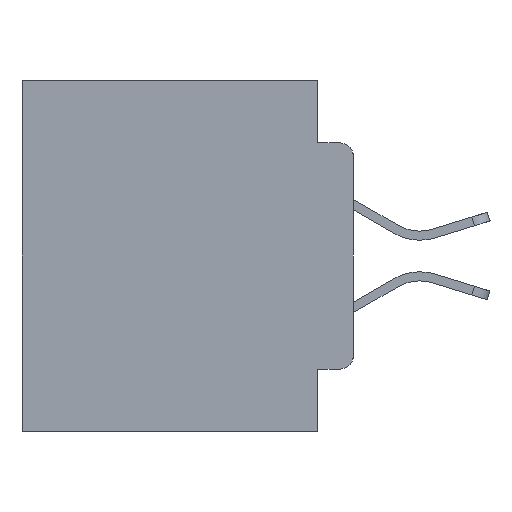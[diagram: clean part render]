
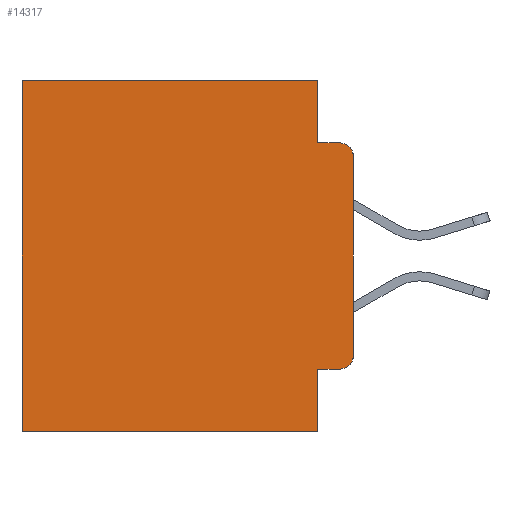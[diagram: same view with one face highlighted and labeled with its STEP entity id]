
A CAD part, left-side view. The second image highlights one B-rep face of the part: STEP entity #14317.
In plain terms, the highlighted planar face has unit normal (-1, 0, 0).
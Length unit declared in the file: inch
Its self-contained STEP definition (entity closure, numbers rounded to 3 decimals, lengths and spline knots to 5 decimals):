
#11 = DIRECTION ( 'NONE',  ( 0., -1., 0. ) ) ;
#180 = EDGE_CURVE ( 'NONE', #10233, #14996, #1160, .T. ) ;
#292 = DIRECTION ( 'NONE',  ( 0., -1., 0. ) ) ;
#867 = LINE ( 'NONE', #10443, #5793 ) ;
#1045 = ORIENTED_EDGE ( 'NONE', *, *, #18575, .F. ) ;
#1160 = LINE ( 'NONE', #14330, #7426 ) ;
#1715 = CARTESIAN_POINT ( 'NONE',  ( 0.298, 0., -0.3915 ) ) ;
#1781 = VECTOR ( 'NONE', #10730, 39.37008 ) ;
#1983 = PLANE ( 'NONE',  #9434 ) ;
#2389 = CARTESIAN_POINT ( 'NONE',  ( 0.298, 0.02, -0.1085 ) ) ;
#2876 = VERTEX_POINT ( 'NONE', #13239 ) ;
#3008 = EDGE_CURVE ( 'NONE', #16063, #8864, #10529, .T. ) ;
#3154 = ORIENTED_EDGE ( 'NONE', *, *, #12785, .F. ) ;
#3588 = AXIS2_PLACEMENT_3D ( 'NONE', #20875, #8948, #22816 ) ;
#4465 = DIRECTION ( 'NONE',  ( 0., 0., -1. ) ) ;
#4980 = LINE ( 'NONE', #25865, #25552 ) ;
#5456 = VERTEX_POINT ( 'NONE', #16748 ) ;
#5793 = VECTOR ( 'NONE', #11, 39.37008 ) ;
#5904 = FACE_OUTER_BOUND ( 'NONE', #18504, .T. ) ;
#6209 = DIRECTION ( 'NONE',  ( 1., 0., 0. ) ) ;
#6647 = CARTESIAN_POINT ( 'NONE',  ( 0.298, 0., -0.1085 ) ) ;
#7142 = ORIENTED_EDGE ( 'NONE', *, *, #14730, .F. ) ;
#7385 = EDGE_CURVE ( 'NONE', #23375, #14602, #9336, .T. ) ;
#7426 = VECTOR ( 'NONE', #9714, 39.37008 ) ;
#7862 = CARTESIAN_POINT ( 'NONE',  ( 0.298, 0.051, 0. ) ) ;
#8667 = CARTESIAN_POINT ( 'NONE',  ( 0.298, 0.051, -0.0885 ) ) ;
#8702 = CARTESIAN_POINT ( 'NONE',  ( 0.298, 0., 0. ) ) ;
#8864 = VERTEX_POINT ( 'NONE', #9341 ) ;
#8948 = DIRECTION ( 'NONE',  ( -1., 0., 0. ) ) ;
#8970 = LINE ( 'NONE', #8667, #19015 ) ;
#9336 = CIRCLE ( 'NONE', #18725, 0.02 ) ;
#9341 = CARTESIAN_POINT ( 'NONE',  ( 0.298, 0.473, -0.5 ) ) ;
#9434 = AXIS2_PLACEMENT_3D ( 'NONE', #18357, #6209, #20303 ) ;
#9667 = ORIENTED_EDGE ( 'NONE', *, *, #20681, .T. ) ;
#9714 = DIRECTION ( 'NONE',  ( 0., 0., -1. ) ) ;
#9991 = EDGE_CURVE ( 'NONE', #2876, #24750, #14282, .T. ) ;
#10041 = ORIENTED_EDGE ( 'NONE', *, *, #9991, .F. ) ;
#10123 = ORIENTED_EDGE ( 'NONE', *, *, #180, .F. ) ;
#10233 = VERTEX_POINT ( 'NONE', #7862 ) ;
#10443 = CARTESIAN_POINT ( 'NONE',  ( 0.298, 0.051, -0.4115 ) ) ;
#10529 = LINE ( 'NONE', #21386, #11164 ) ;
#10730 = DIRECTION ( 'NONE',  ( 0., 1., 0. ) ) ;
#11164 = VECTOR ( 'NONE', #14264, 39.37008 ) ;
#12785 = EDGE_CURVE ( 'NONE', #24750, #8864, #4980, .T. ) ;
#13239 = CARTESIAN_POINT ( 'NONE',  ( 0.298, 0.051, -0.4115 ) ) ;
#13597 = ORIENTED_EDGE ( 'NONE', *, *, #16756, .T. ) ;
#14264 = DIRECTION ( 'NONE',  ( 0., 0., -1. ) ) ;
#14282 = LINE ( 'NONE', #14794, #18316 ) ;
#14317 = ADVANCED_FACE ( 'NONE', ( #5904 ), #1983, .F. ) ;
#14330 = CARTESIAN_POINT ( 'NONE',  ( 0.298, 0.051, 0. ) ) ;
#14602 = VERTEX_POINT ( 'NONE', #23064 ) ;
#14730 = EDGE_CURVE ( 'NONE', #23375, #16025, #17338, .T. ) ;
#14794 = CARTESIAN_POINT ( 'NONE',  ( 0.298, 0.051, 0. ) ) ;
#14996 = VERTEX_POINT ( 'NONE', #25937 ) ;
#15062 = CARTESIAN_POINT ( 'NONE',  ( 0.298, 0.051, -0.5 ) ) ;
#15657 = CARTESIAN_POINT ( 'NONE',  ( 0.298, 0., 0. ) ) ;
#16025 = VERTEX_POINT ( 'NONE', #1715 ) ;
#16063 = VERTEX_POINT ( 'NONE', #18101 ) ;
#16729 = VECTOR ( 'NONE', #25299, 39.37008 ) ;
#16748 = CARTESIAN_POINT ( 'NONE',  ( 0.298, 0.02, -0.4115 ) ) ;
#16754 = DIRECTION ( 'NONE',  ( -1., 0., 0. ) ) ;
#16756 = EDGE_CURVE ( 'NONE', #2876, #5456, #867, .T. ) ;
#17338 = LINE ( 'NONE', #15657, #16729 ) ;
#17623 = ORIENTED_EDGE ( 'NONE', *, *, #7385, .T. ) ;
#17948 = EDGE_CURVE ( 'NONE', #10233, #16063, #18244, .T. ) ;
#18101 = CARTESIAN_POINT ( 'NONE',  ( 0.298, 0.473, 0. ) ) ;
#18243 = DIRECTION ( 'NONE',  ( 0., 1., 0. ) ) ;
#18244 = LINE ( 'NONE', #8702, #1781 ) ;
#18316 = VECTOR ( 'NONE', #24490, 39.37008 ) ;
#18357 = CARTESIAN_POINT ( 'NONE',  ( 0.298, 0., 0. ) ) ;
#18504 = EDGE_LOOP ( 'NONE', ( #7142, #17623, #1045, #10123, #24891, #21851, #3154, #10041, #13597, #9667 ) ) ;
#18575 = EDGE_CURVE ( 'NONE', #14996, #14602, #8970, .T. ) ;
#18725 = AXIS2_PLACEMENT_3D ( 'NONE', #2389, #16754, #4465 ) ;
#19015 = VECTOR ( 'NONE', #292, 39.37008 ) ;
#20303 = DIRECTION ( 'NONE',  ( 0., 0., -1. ) ) ;
#20681 = EDGE_CURVE ( 'NONE', #5456, #16025, #21283, .T. ) ;
#20875 = CARTESIAN_POINT ( 'NONE',  ( 0.298, 0.02, -0.3915 ) ) ;
#21283 = CIRCLE ( 'NONE', #3588, 0.02 ) ;
#21386 = CARTESIAN_POINT ( 'NONE',  ( 0.298, 0.473, 0. ) ) ;
#21851 = ORIENTED_EDGE ( 'NONE', *, *, #3008, .T. ) ;
#22816 = DIRECTION ( 'NONE',  ( 0., 0., -1. ) ) ;
#23064 = CARTESIAN_POINT ( 'NONE',  ( 0.298, 0.02, -0.0885 ) ) ;
#23375 = VERTEX_POINT ( 'NONE', #6647 ) ;
#24490 = DIRECTION ( 'NONE',  ( 0., 0., -1. ) ) ;
#24750 = VERTEX_POINT ( 'NONE', #15062 ) ;
#24891 = ORIENTED_EDGE ( 'NONE', *, *, #17948, .T. ) ;
#25299 = DIRECTION ( 'NONE',  ( 0., 0., -1. ) ) ;
#25552 = VECTOR ( 'NONE', #18243, 39.37008 ) ;
#25865 = CARTESIAN_POINT ( 'NONE',  ( 0.298, 0., -0.5 ) ) ;
#25937 = CARTESIAN_POINT ( 'NONE',  ( 0.298, 0.051, -0.0885 ) ) ;
